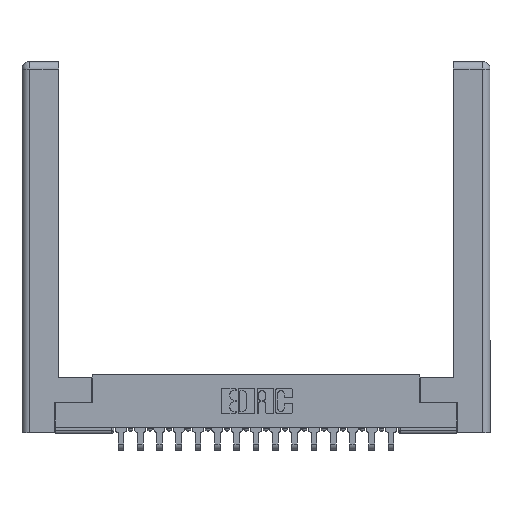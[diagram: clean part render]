
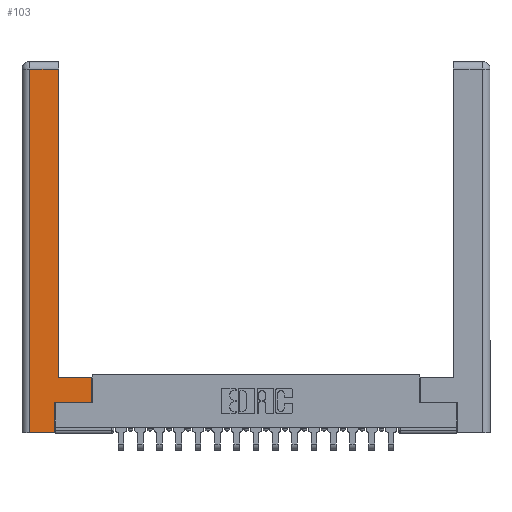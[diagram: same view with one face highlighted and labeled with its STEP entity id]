
A CAD part, top view. The second image highlights one B-rep face of the part: STEP entity #103.
In plain terms, the highlighted planar face has unit normal (0, 0, 1).
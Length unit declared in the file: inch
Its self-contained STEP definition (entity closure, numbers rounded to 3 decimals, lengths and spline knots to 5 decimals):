
#103 = ADVANCED_FACE ( 'NONE', ( #7646 ), #8560, .F. ) ;
#181 = CARTESIAN_POINT ( 'NONE',  ( 0.295, 3., 0. ) ) ;
#387 = ORIENTED_EDGE ( 'NONE', *, *, #17994, .T. ) ;
#527 = VECTOR ( 'NONE', #13613, 39.37008 ) ;
#535 = VERTEX_POINT ( 'NONE', #4274 ) ;
#1700 = VECTOR ( 'NONE', #2182, 39.37008 ) ;
#1799 = VECTOR ( 'NONE', #2769, 39.37008 ) ;
#1808 = VECTOR ( 'NONE', #6815, 39.37008 ) ;
#1916 = CARTESIAN_POINT ( 'NONE',  ( 0.0615, 2.94, 0. ) ) ;
#1932 = ORIENTED_EDGE ( 'NONE', *, *, #14106, .T. ) ;
#2152 = ORIENTED_EDGE ( 'NONE', *, *, #6308, .T. ) ;
#2182 = DIRECTION ( 'NONE',  ( 1., 0., 0. ) ) ;
#2495 = CARTESIAN_POINT ( 'NONE',  ( 0.265, 0., 0. ) ) ;
#2723 = DIRECTION ( 'NONE',  ( -1., 0., 0. ) ) ;
#2769 = DIRECTION ( 'NONE',  ( 0., 1., 0. ) ) ;
#2862 = DIRECTION ( 'NONE',  ( 0., 1., 0. ) ) ;
#3135 = CARTESIAN_POINT ( 'NONE',  ( 0.295, 0.45, 0. ) ) ;
#3169 = CARTESIAN_POINT ( 'NONE',  ( 0.0615, 0., 0. ) ) ;
#3319 = ORIENTED_EDGE ( 'NONE', *, *, #4371, .T. ) ;
#3609 = VECTOR ( 'NONE', #2862, 39.37008 ) ;
#4274 = CARTESIAN_POINT ( 'NONE',  ( 0.295, 0.45, 0. ) ) ;
#4281 = VERTEX_POINT ( 'NONE', #5387 ) ;
#4293 = LINE ( 'NONE', #3135, #8881 ) ;
#4331 = CARTESIAN_POINT ( 'NONE',  ( 0.0615, 2.94, 0. ) ) ;
#4371 = EDGE_CURVE ( 'NONE', #4281, #13229, #8173, .T. ) ;
#5204 = CARTESIAN_POINT ( 'NONE',  ( 0.565, 0.245, 0. ) ) ;
#5387 = CARTESIAN_POINT ( 'NONE',  ( 0.565, 0.245, 0. ) ) ;
#5411 = VECTOR ( 'NONE', #18588, 39.37008 ) ;
#5632 = DIRECTION ( 'NONE',  ( 0., 0., -1. ) ) ;
#5865 = VERTEX_POINT ( 'NONE', #6431 ) ;
#5876 = EDGE_CURVE ( 'NONE', #5865, #4281, #15387, .T. ) ;
#5963 = LINE ( 'NONE', #181, #17347 ) ;
#6308 = EDGE_CURVE ( 'NONE', #535, #7252, #5963, .T. ) ;
#6431 = CARTESIAN_POINT ( 'NONE',  ( 0.265, 0.245, 0. ) ) ;
#6815 = DIRECTION ( 'NONE',  ( 0., -1., 0. ) ) ;
#6886 = EDGE_CURVE ( 'NONE', #14562, #5865, #17796, .T. ) ;
#7252 = VERTEX_POINT ( 'NONE', #8080 ) ;
#7646 = FACE_OUTER_BOUND ( 'NONE', #7816, .T. ) ;
#7706 = EDGE_CURVE ( 'NONE', #13229, #535, #4293, .T. ) ;
#7816 = EDGE_LOOP ( 'NONE', ( #2152, #387, #1932, #7935, #10286, #9891, #3319, #11180 ) ) ;
#7935 = ORIENTED_EDGE ( 'NONE', *, *, #15894, .T. ) ;
#8080 = CARTESIAN_POINT ( 'NONE',  ( 0.295, 2.94, 0. ) ) ;
#8173 = LINE ( 'NONE', #17538, #3609 ) ;
#8337 = CARTESIAN_POINT ( 'NONE',  ( 0.0615, 0., 0. ) ) ;
#8560 = PLANE ( 'NONE',  #16936 ) ;
#8881 = VECTOR ( 'NONE', #16279, 39.37008 ) ;
#9364 = LINE ( 'NONE', #8337, #1808 ) ;
#9465 = VERTEX_POINT ( 'NONE', #3169 ) ;
#9891 = ORIENTED_EDGE ( 'NONE', *, *, #5876, .T. ) ;
#9997 = CARTESIAN_POINT ( 'NONE',  ( 0.265, 0.245, 0. ) ) ;
#10286 = ORIENTED_EDGE ( 'NONE', *, *, #6886, .T. ) ;
#11180 = ORIENTED_EDGE ( 'NONE', *, *, #7706, .T. ) ;
#11476 = CARTESIAN_POINT ( 'NONE',  ( 0., 0., 0. ) ) ;
#11871 = CARTESIAN_POINT ( 'NONE',  ( 0.565, 0.45, 0. ) ) ;
#13120 = LINE ( 'NONE', #1916, #527 ) ;
#13229 = VERTEX_POINT ( 'NONE', #11871 ) ;
#13553 = CARTESIAN_POINT ( 'NONE',  ( 0.265, 0., 0. ) ) ;
#13613 = DIRECTION ( 'NONE',  ( -1., 0., 0. ) ) ;
#14106 = EDGE_CURVE ( 'NONE', #14924, #9465, #9364, .T. ) ;
#14562 = VERTEX_POINT ( 'NONE', #13553 ) ;
#14924 = VERTEX_POINT ( 'NONE', #4331 ) ;
#15387 = LINE ( 'NONE', #5204, #1700 ) ;
#15894 = EDGE_CURVE ( 'NONE', #9465, #14562, #18199, .T. ) ;
#16132 = DIRECTION ( 'NONE',  ( 0., 1., 0. ) ) ;
#16279 = DIRECTION ( 'NONE',  ( -1., 0., 0. ) ) ;
#16936 = AXIS2_PLACEMENT_3D ( 'NONE', #11476, #5632, #2723 ) ;
#17347 = VECTOR ( 'NONE', #16132, 39.37008 ) ;
#17538 = CARTESIAN_POINT ( 'NONE',  ( 0.565, 0.45, 0. ) ) ;
#17796 = LINE ( 'NONE', #9997, #1799 ) ;
#17994 = EDGE_CURVE ( 'NONE', #7252, #14924, #13120, .T. ) ;
#18199 = LINE ( 'NONE', #2495, #5411 ) ;
#18588 = DIRECTION ( 'NONE',  ( 1., 0., 0. ) ) ;
